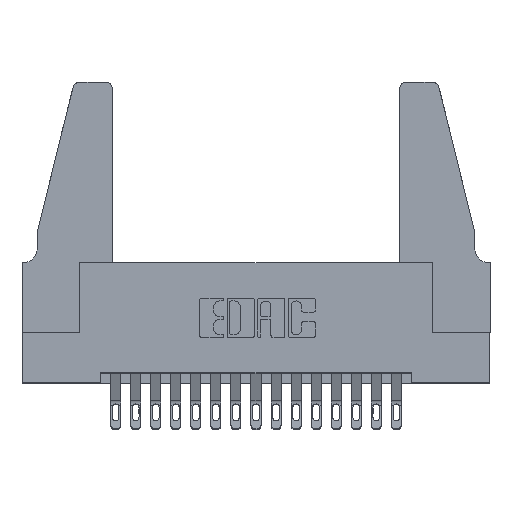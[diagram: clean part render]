
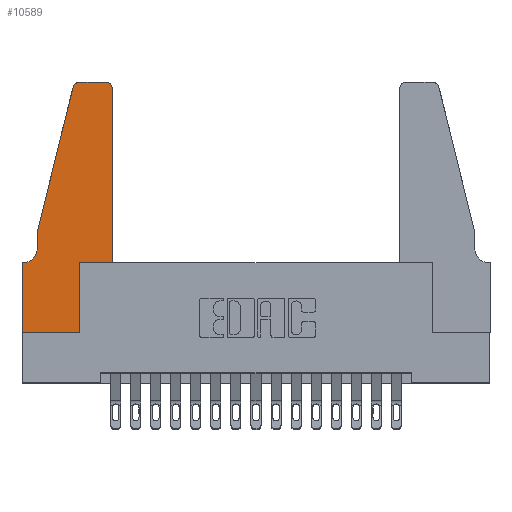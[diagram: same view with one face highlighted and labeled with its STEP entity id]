
A CAD part, top view. The second image highlights one B-rep face of the part: STEP entity #10589.
In plain terms, the highlighted planar face has unit normal (0, 0, 1).
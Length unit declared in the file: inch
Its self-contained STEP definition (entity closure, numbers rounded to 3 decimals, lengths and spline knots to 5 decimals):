
#208 = VERTEX_POINT ( 'NONE', #14769 ) ;
#404 = AXIS2_PLACEMENT_3D ( 'NONE', #5845, #1606, #7185 ) ;
#524 = VERTEX_POINT ( 'NONE', #1414 ) ;
#561 = CARTESIAN_POINT ( 'NONE',  ( 0.4505, 0.35, 0.37 ) ) ;
#586 = CARTESIAN_POINT ( 'NONE',  ( 0.284, 1.22, 0.37 ) ) ;
#686 = EDGE_CURVE ( 'NONE', #10231, #4945, #979, .T. ) ;
#695 = DIRECTION ( 'NONE',  ( 0., 1., 0. ) ) ;
#979 = LINE ( 'NONE', #6056, #7913 ) ;
#1319 = ORIENTED_EDGE ( 'NONE', *, *, #2882, .T. ) ;
#1414 = CARTESIAN_POINT ( 'NONE',  ( 0.0755, 0.5, 0.37 ) ) ;
#1606 = DIRECTION ( 'NONE',  ( 0., 0., 1. ) ) ;
#1792 = DIRECTION ( 'NONE',  ( -0.239, -0.971, 0. ) ) ;
#1825 = EDGE_CURVE ( 'NONE', #208, #524, #10450, .T. ) ;
#1875 = ORIENTED_EDGE ( 'NONE', *, *, #10247, .T. ) ;
#1929 = EDGE_CURVE ( 'NONE', #14428, #7730, #6790, .T. ) ;
#2008 = VERTEX_POINT ( 'NONE', #13039 ) ;
#2254 = CARTESIAN_POINT ( 'NONE',  ( 0.4205, 1.25, 0.37 ) ) ;
#2370 = FACE_OUTER_BOUND ( 'NONE', #7556, .T. ) ;
#2385 = LINE ( 'NONE', #9659, #7789 ) ;
#2548 = ORIENTED_EDGE ( 'NONE', *, *, #13677, .T. ) ;
#2837 = VERTEX_POINT ( 'NONE', #12650 ) ;
#2882 = EDGE_CURVE ( 'NONE', #2837, #10231, #17766, .T. ) ;
#2899 = VECTOR ( 'NONE', #9708, 39.37008 ) ;
#3159 = EDGE_CURVE ( 'NONE', #14078, #2837, #13243, .T. ) ;
#3691 = DIRECTION ( 'NONE',  ( -1., 0., 0. ) ) ;
#3861 = ORIENTED_EDGE ( 'NONE', *, *, #686, .T. ) ;
#4770 = ORIENTED_EDGE ( 'NONE', *, *, #8320, .T. ) ;
#4905 = DIRECTION ( 'NONE',  ( 1., 0., 0. ) ) ;
#4945 = VERTEX_POINT ( 'NONE', #7916 ) ;
#5429 = AXIS2_PLACEMENT_3D ( 'NONE', #586, #13236, #11653 ) ;
#5522 = VERTEX_POINT ( 'NONE', #14693 ) ;
#5845 = CARTESIAN_POINT ( 'NONE',  ( 0.4205, 1.22, 0.37 ) ) ;
#6056 = CARTESIAN_POINT ( 'NONE',  ( 0., 0., 0.37 ) ) ;
#6624 = DIRECTION ( 'NONE',  ( -1., 0., 0. ) ) ;
#6684 = DIRECTION ( 'NONE',  ( 0., -1., 0. ) ) ;
#6790 = LINE ( 'NONE', #561, #15809 ) ;
#7158 = CIRCLE ( 'NONE', #15338, 0.07 ) ;
#7185 = DIRECTION ( 'NONE',  ( 1., 0., 0. ) ) ;
#7285 = ORIENTED_EDGE ( 'NONE', *, *, #16976, .T. ) ;
#7556 = EDGE_LOOP ( 'NONE', ( #12675, #7285, #15831, #2548, #16715, #11268, #1319, #3861, #4770, #1875, #16579, #10404 ) ) ;
#7730 = VERTEX_POINT ( 'NONE', #11574 ) ;
#7789 = VECTOR ( 'NONE', #8163, 39.37008 ) ;
#7913 = VECTOR ( 'NONE', #4905, 39.37008 ) ;
#7916 = CARTESIAN_POINT ( 'NONE',  ( 0.2865, 0., 0.37 ) ) ;
#8042 = DIRECTION ( 'NONE',  ( 0., 1., 0. ) ) ;
#8131 = LINE ( 'NONE', #14948, #11993 ) ;
#8163 = DIRECTION ( 'NONE',  ( 1., 0., 0. ) ) ;
#8237 = CARTESIAN_POINT ( 'NONE',  ( 0.284, 1.25, 0.37 ) ) ;
#8303 = CARTESIAN_POINT ( 'NONE',  ( 0.4505, 0.35, 0.37 ) ) ;
#8320 = EDGE_CURVE ( 'NONE', #4945, #2008, #10292, .T. ) ;
#8766 = CARTESIAN_POINT ( 'NONE',  ( 0.0055, 0.35, 0.37 ) ) ;
#8877 = CIRCLE ( 'NONE', #404, 0.03 ) ;
#9138 = PLANE ( 'NONE',  #15961 ) ;
#9143 = CIRCLE ( 'NONE', #5429, 0.03 ) ;
#9597 = CARTESIAN_POINT ( 'NONE',  ( 0.2865, 0.35, 0.37 ) ) ;
#9659 = CARTESIAN_POINT ( 'NONE',  ( 0.4505, 0.35, 0.37 ) ) ;
#9708 = DIRECTION ( 'NONE',  ( -1., 0., 0. ) ) ;
#9942 = CARTESIAN_POINT ( 'NONE',  ( 0.2605, 1.25, 0.37 ) ) ;
#10231 = VERTEX_POINT ( 'NONE', #12491 ) ;
#10247 = EDGE_CURVE ( 'NONE', #2008, #14428, #2385, .T. ) ;
#10292 = LINE ( 'NONE', #9597, #17194 ) ;
#10342 = DIRECTION ( 'NONE',  ( 0., -1., 0. ) ) ;
#10404 = ORIENTED_EDGE ( 'NONE', *, *, #16042, .T. ) ;
#10450 = LINE ( 'NONE', #16756, #11728 ) ;
#10514 = CARTESIAN_POINT ( 'NONE',  ( 0.0755, 0.35, 0.37 ) ) ;
#10589 = ADVANCED_FACE ( 'NONE', ( #2370 ), #9138, .T. ) ;
#11268 = ORIENTED_EDGE ( 'NONE', *, *, #3159, .T. ) ;
#11484 = VERTEX_POINT ( 'NONE', #8237 ) ;
#11574 = CARTESIAN_POINT ( 'NONE',  ( 0.4505, 1.22, 0.37 ) ) ;
#11608 = CARTESIAN_POINT ( 'NONE',  ( 0., 0., 0.37 ) ) ;
#11653 = DIRECTION ( 'NONE',  ( 1., 0., 0. ) ) ;
#11728 = VECTOR ( 'NONE', #1792, 39.37008 ) ;
#11993 = VECTOR ( 'NONE', #6684, 39.37008 ) ;
#12348 = DIRECTION ( 'NONE',  ( 0., 0., -1. ) ) ;
#12409 = LINE ( 'NONE', #9942, #2899 ) ;
#12491 = CARTESIAN_POINT ( 'NONE',  ( 0., 0., 0.37 ) ) ;
#12602 = VECTOR ( 'NONE', #10342, 39.37008 ) ;
#12650 = CARTESIAN_POINT ( 'NONE',  ( 0., 0.35, 0.37 ) ) ;
#12675 = ORIENTED_EDGE ( 'NONE', *, *, #16654, .T. ) ;
#13039 = CARTESIAN_POINT ( 'NONE',  ( 0.2865, 0.35, 0.37 ) ) ;
#13192 = CARTESIAN_POINT ( 'NONE',  ( 0., 0.35, 0.37 ) ) ;
#13236 = DIRECTION ( 'NONE',  ( 0., 0., 1. ) ) ;
#13243 = LINE ( 'NONE', #10514, #17097 ) ;
#13677 = EDGE_CURVE ( 'NONE', #524, #5522, #8131, .T. ) ;
#14078 = VERTEX_POINT ( 'NONE', #8766 ) ;
#14298 = VERTEX_POINT ( 'NONE', #2254 ) ;
#14428 = VERTEX_POINT ( 'NONE', #8303 ) ;
#14693 = CARTESIAN_POINT ( 'NONE',  ( 0.0755, 0.42, 0.37 ) ) ;
#14769 = CARTESIAN_POINT ( 'NONE',  ( 0.25487, 1.22718, 0.37 ) ) ;
#14948 = CARTESIAN_POINT ( 'NONE',  ( 0.0755, 0.5, 0.37 ) ) ;
#15338 = AXIS2_PLACEMENT_3D ( 'NONE', #17896, #12348, #6624 ) ;
#15809 = VECTOR ( 'NONE', #695, 39.37008 ) ;
#15831 = ORIENTED_EDGE ( 'NONE', *, *, #1825, .T. ) ;
#15961 = AXIS2_PLACEMENT_3D ( 'NONE', #13192, #17477, #17280 ) ;
#16042 = EDGE_CURVE ( 'NONE', #7730, #14298, #8877, .T. ) ;
#16448 = EDGE_CURVE ( 'NONE', #5522, #14078, #7158, .T. ) ;
#16579 = ORIENTED_EDGE ( 'NONE', *, *, #1929, .T. ) ;
#16654 = EDGE_CURVE ( 'NONE', #14298, #11484, #12409, .T. ) ;
#16715 = ORIENTED_EDGE ( 'NONE', *, *, #16448, .T. ) ;
#16756 = CARTESIAN_POINT ( 'NONE',  ( 0.0755, 0.5, 0.37 ) ) ;
#16976 = EDGE_CURVE ( 'NONE', #11484, #208, #9143, .T. ) ;
#17097 = VECTOR ( 'NONE', #3691, 39.37008 ) ;
#17194 = VECTOR ( 'NONE', #8042, 39.37008 ) ;
#17280 = DIRECTION ( 'NONE',  ( 1., 0., 0. ) ) ;
#17477 = DIRECTION ( 'NONE',  ( 0., 0., 1. ) ) ;
#17766 = LINE ( 'NONE', #11608, #12602 ) ;
#17896 = CARTESIAN_POINT ( 'NONE',  ( 0.0055, 0.42, 0.37 ) ) ;
